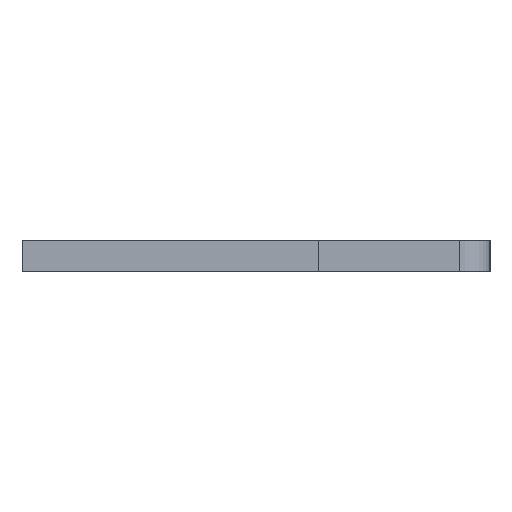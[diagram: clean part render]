
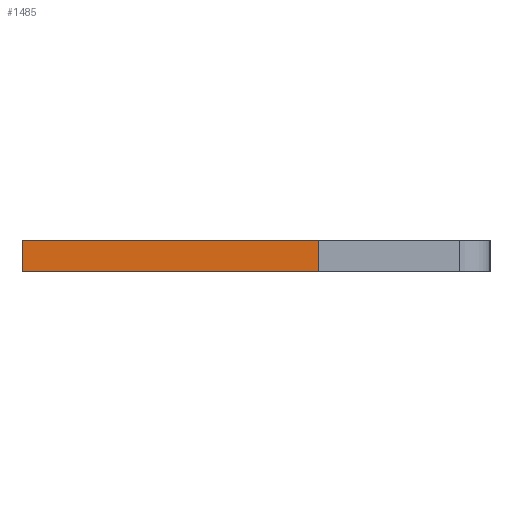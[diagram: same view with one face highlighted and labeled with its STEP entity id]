
A CAD part, left-side view. The second image highlights one B-rep face of the part: STEP entity #1485.
In plain terms, the highlighted face is planar.
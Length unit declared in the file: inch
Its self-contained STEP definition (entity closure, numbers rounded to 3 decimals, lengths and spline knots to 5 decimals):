
#33 = ORIENTED_EDGE ( 'NONE', *, *, #1112, .F. ) ;
#35 = VECTOR ( 'NONE', #735, 39.37008 ) ;
#77 = LINE ( 'NONE', #1164, #35 ) ;
#127 = VERTEX_POINT ( 'NONE', #243 ) ;
#131 = DIRECTION ( 'NONE',  ( -1., 0., 0. ) ) ;
#142 = DIRECTION ( 'NONE',  ( 0., 1., 0. ) ) ;
#156 = CARTESIAN_POINT ( 'NONE',  ( -0.01, 0.15, -0.04 ) ) ;
#226 = CARTESIAN_POINT ( 'NONE',  ( 0.01, 0.15, -0.04 ) ) ;
#237 = LINE ( 'NONE', #1368, #1502 ) ;
#243 = CARTESIAN_POINT ( 'NONE',  ( -0.01, -0.04, -0.04 ) ) ;
#263 = CARTESIAN_POINT ( 'NONE',  ( -0.01, 0.15, -0.04 ) ) ;
#360 = ORIENTED_EDGE ( 'NONE', *, *, #403, .F. ) ;
#403 = EDGE_CURVE ( 'NONE', #1068, #1474, #887, .T. ) ;
#433 = CARTESIAN_POINT ( 'NONE',  ( 0.01, -0.04, -0.04 ) ) ;
#639 = VECTOR ( 'NONE', #1564, 39.37008 ) ;
#662 = VERTEX_POINT ( 'NONE', #263 ) ;
#685 = EDGE_CURVE ( 'NONE', #1068, #127, #237, .T. ) ;
#735 = DIRECTION ( 'NONE',  ( -1., 0., 0. ) ) ;
#760 = CARTESIAN_POINT ( 'NONE',  ( 0.01, 0.15, -0.04 ) ) ;
#781 = DIRECTION ( 'NONE',  ( 0., 0., 1. ) ) ;
#864 = LINE ( 'NONE', #156, #639 ) ;
#887 = LINE ( 'NONE', #1393, #1584 ) ;
#965 = EDGE_CURVE ( 'NONE', #127, #662, #864, .T. ) ;
#1004 = ORIENTED_EDGE ( 'NONE', *, *, #685, .T. ) ;
#1065 = ORIENTED_EDGE ( 'NONE', *, *, #965, .T. ) ;
#1068 = VERTEX_POINT ( 'NONE', #433 ) ;
#1112 = EDGE_CURVE ( 'NONE', #1474, #662, #77, .T. ) ;
#1121 = FACE_OUTER_BOUND ( 'NONE', #1647, .T. ) ;
#1164 = CARTESIAN_POINT ( 'NONE',  ( 0.01, 0.15, -0.04 ) ) ;
#1332 = PLANE ( 'NONE',  #1776 ) ;
#1368 = CARTESIAN_POINT ( 'NONE',  ( 0.01, -0.04, -0.04 ) ) ;
#1393 = CARTESIAN_POINT ( 'NONE',  ( 0.01, 0.15, -0.04 ) ) ;
#1474 = VERTEX_POINT ( 'NONE', #760 ) ;
#1485 = ADVANCED_FACE ( 'NONE', ( #1121 ), #1332, .F. ) ;
#1502 = VECTOR ( 'NONE', #131, 39.37008 ) ;
#1564 = DIRECTION ( 'NONE',  ( 0., 1., 0. ) ) ;
#1584 = VECTOR ( 'NONE', #142, 39.37008 ) ;
#1647 = EDGE_LOOP ( 'NONE', ( #1065, #33, #360, #1004 ) ) ;
#1750 = DIRECTION ( 'NONE',  ( 1., 0., 0. ) ) ;
#1776 = AXIS2_PLACEMENT_3D ( 'NONE', #226, #781, #1750 ) ;
